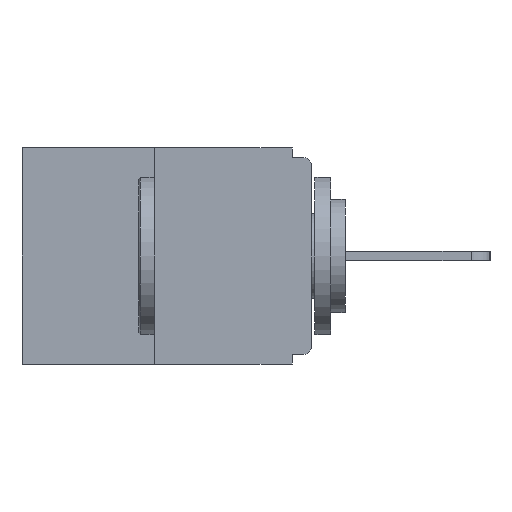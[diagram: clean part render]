
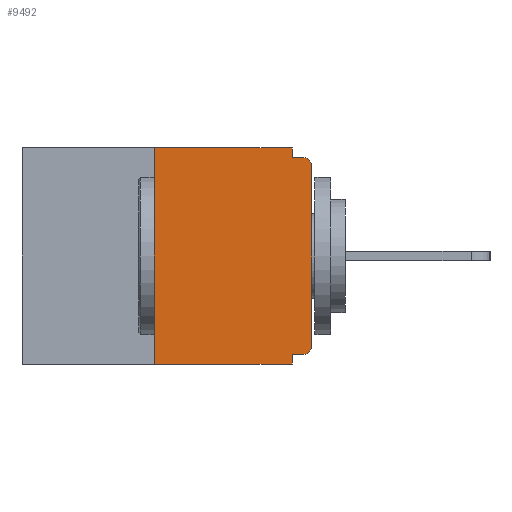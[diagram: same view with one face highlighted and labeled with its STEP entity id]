
A CAD part, left-side view. The second image highlights one B-rep face of the part: STEP entity #9492.
In plain terms, the highlighted planar face has unit normal (-1, 0, 0).
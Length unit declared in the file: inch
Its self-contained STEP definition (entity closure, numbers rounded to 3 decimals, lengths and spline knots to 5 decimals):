
#80 = DIRECTION ( 'NONE',  ( -1., 0., 0. ) ) ;
#112 = VERTEX_POINT ( 'NONE', #7646 ) ;
#189 = CARTESIAN_POINT ( 'NONE',  ( 0., 0.031, -0.343 ) ) ;
#349 = FACE_OUTER_BOUND ( 'NONE', #11585, .T. ) ;
#870 = DIRECTION ( 'NONE',  ( 0., 0., -1. ) ) ;
#1086 = EDGE_CURVE ( 'NONE', #6322, #112, #20432, .T. ) ;
#1744 = ORIENTED_EDGE ( 'NONE', *, *, #13876, .T. ) ;
#1957 = CARTESIAN_POINT ( 'NONE',  ( 0., 0.031, -0.343 ) ) ;
#2063 = DIRECTION ( 'NONE',  ( 1., 0., 0. ) ) ;
#2167 = DIRECTION ( 'NONE',  ( 0., 0., -1. ) ) ;
#2365 = DIRECTION ( 'NONE',  ( -1., 0., 0. ) ) ;
#2991 = VECTOR ( 'NONE', #18181, 39.37008 ) ;
#3182 = CARTESIAN_POINT ( 'NONE',  ( 0., 0.031, -0.015 ) ) ;
#3516 = VECTOR ( 'NONE', #14010, 39.37008 ) ;
#3551 = VECTOR ( 'NONE', #8938, 39.37008 ) ;
#3689 = LINE ( 'NONE', #6663, #20528 ) ;
#3915 = AXIS2_PLACEMENT_3D ( 'NONE', #10403, #2063, #2167 ) ;
#3996 = VERTEX_POINT ( 'NONE', #1957 ) ;
#4565 = CARTESIAN_POINT ( 'NONE',  ( 0., 0.25, 0. ) ) ;
#4865 = VECTOR ( 'NONE', #10034, 39.37008 ) ;
#5031 = VECTOR ( 'NONE', #870, 39.37008 ) ;
#5149 = CARTESIAN_POINT ( 'NONE',  ( 0., 0., 0. ) ) ;
#5258 = EDGE_CURVE ( 'NONE', #7256, #10112, #3689, .T. ) ;
#5425 = ORIENTED_EDGE ( 'NONE', *, *, #13135, .F. ) ;
#5571 = CIRCLE ( 'NONE', #7960, 0.015 ) ;
#5891 = ORIENTED_EDGE ( 'NONE', *, *, #6086, .F. ) ;
#5977 = VERTEX_POINT ( 'NONE', #14852 ) ;
#6086 = EDGE_CURVE ( 'NONE', #5977, #3996, #9930, .T. ) ;
#6201 = CARTESIAN_POINT ( 'NONE',  ( 0., 0.031, 0. ) ) ;
#6322 = VERTEX_POINT ( 'NONE', #16083 ) ;
#6663 = CARTESIAN_POINT ( 'NONE',  ( 0., 0.25, 0. ) ) ;
#7256 = VERTEX_POINT ( 'NONE', #11747 ) ;
#7578 = ORIENTED_EDGE ( 'NONE', *, *, #8178, .F. ) ;
#7646 = CARTESIAN_POINT ( 'NONE',  ( 0., 0.015, -0.015 ) ) ;
#7878 = EDGE_CURVE ( 'NONE', #7256, #3996, #20853, .T. ) ;
#7960 = AXIS2_PLACEMENT_3D ( 'NONE', #14746, #80, #9331 ) ;
#8178 = EDGE_CURVE ( 'NONE', #14679, #112, #12197, .T. ) ;
#8440 = CARTESIAN_POINT ( 'NONE',  ( 0., 0.031, 0. ) ) ;
#8482 = VERTEX_POINT ( 'NONE', #9713 ) ;
#8584 = ORIENTED_EDGE ( 'NONE', *, *, #7878, .T. ) ;
#8897 = DIRECTION ( 'NONE',  ( 0., 0., -1. ) ) ;
#8938 = DIRECTION ( 'NONE',  ( 0., -1., 0. ) ) ;
#8990 = EDGE_CURVE ( 'NONE', #10112, #9738, #11950, .T. ) ;
#9095 = CARTESIAN_POINT ( 'NONE',  ( 0., 0., -0.015 ) ) ;
#9331 = DIRECTION ( 'NONE',  ( 0., 0., -1. ) ) ;
#9337 = ORIENTED_EDGE ( 'NONE', *, *, #16740, .T. ) ;
#9492 = ADVANCED_FACE ( 'NONE', ( #349 ), #20338, .F. ) ;
#9713 = CARTESIAN_POINT ( 'NONE',  ( 0., 0.015, -0.328 ) ) ;
#9738 = VERTEX_POINT ( 'NONE', #8440 ) ;
#9930 = LINE ( 'NONE', #189, #4865 ) ;
#10034 = DIRECTION ( 'NONE',  ( 0., 0., -1. ) ) ;
#10042 = LINE ( 'NONE', #13264, #15306 ) ;
#10112 = VERTEX_POINT ( 'NONE', #4565 ) ;
#10403 = CARTESIAN_POINT ( 'NONE',  ( 0., 0.46, 0. ) ) ;
#10471 = DIRECTION ( 'NONE',  ( 0., 1., 0. ) ) ;
#11239 = CARTESIAN_POINT ( 'NONE',  ( 0., 0., -0.313 ) ) ;
#11377 = DIRECTION ( 'NONE',  ( 0., 0., 1. ) ) ;
#11420 = ORIENTED_EDGE ( 'NONE', *, *, #8990, .F. ) ;
#11585 = EDGE_LOOP ( 'NONE', ( #11420, #16457, #8584, #5891, #5425, #9337, #1744, #20388, #7578, #19207 ) ) ;
#11747 = CARTESIAN_POINT ( 'NONE',  ( 0., 0.25, -0.343 ) ) ;
#11950 = LINE ( 'NONE', #13649, #3551 ) ;
#12197 = LINE ( 'NONE', #9095, #3516 ) ;
#13135 = EDGE_CURVE ( 'NONE', #8482, #5977, #10042, .T. ) ;
#13264 = CARTESIAN_POINT ( 'NONE',  ( 0., 0., -0.328 ) ) ;
#13303 = LINE ( 'NONE', #5149, #2991 ) ;
#13649 = CARTESIAN_POINT ( 'NONE',  ( 0., 0.46, 0. ) ) ;
#13876 = EDGE_CURVE ( 'NONE', #20951, #6322, #13303, .T. ) ;
#13965 = AXIS2_PLACEMENT_3D ( 'NONE', #14231, #2365, #8897 ) ;
#14010 = DIRECTION ( 'NONE',  ( 0., -1., 0. ) ) ;
#14165 = EDGE_CURVE ( 'NONE', #9738, #14679, #14342, .T. ) ;
#14231 = CARTESIAN_POINT ( 'NONE',  ( 0., 0.015, -0.03 ) ) ;
#14342 = LINE ( 'NONE', #6201, #5031 ) ;
#14679 = VERTEX_POINT ( 'NONE', #3182 ) ;
#14746 = CARTESIAN_POINT ( 'NONE',  ( 0., 0.015, -0.313 ) ) ;
#14852 = CARTESIAN_POINT ( 'NONE',  ( 0., 0.031, -0.328 ) ) ;
#15306 = VECTOR ( 'NONE', #10471, 39.37008 ) ;
#15952 = CARTESIAN_POINT ( 'NONE',  ( 0., 0.46, -0.343 ) ) ;
#16083 = CARTESIAN_POINT ( 'NONE',  ( 0., 0., -0.03 ) ) ;
#16457 = ORIENTED_EDGE ( 'NONE', *, *, #5258, .F. ) ;
#16740 = EDGE_CURVE ( 'NONE', #8482, #20951, #5571, .T. ) ;
#17843 = DIRECTION ( 'NONE',  ( 0., -1., 0. ) ) ;
#18181 = DIRECTION ( 'NONE',  ( 0., 0., 1. ) ) ;
#19207 = ORIENTED_EDGE ( 'NONE', *, *, #14165, .F. ) ;
#20272 = VECTOR ( 'NONE', #17843, 39.37008 ) ;
#20338 = PLANE ( 'NONE',  #3915 ) ;
#20388 = ORIENTED_EDGE ( 'NONE', *, *, #1086, .T. ) ;
#20432 = CIRCLE ( 'NONE', #13965, 0.015 ) ;
#20528 = VECTOR ( 'NONE', #11377, 39.37008 ) ;
#20853 = LINE ( 'NONE', #15952, #20272 ) ;
#20951 = VERTEX_POINT ( 'NONE', #11239 ) ;
